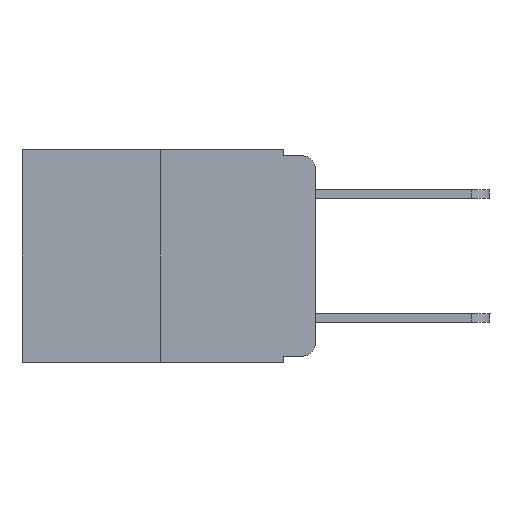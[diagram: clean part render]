
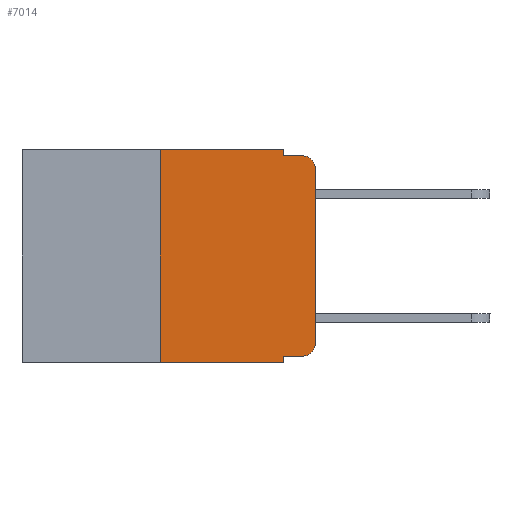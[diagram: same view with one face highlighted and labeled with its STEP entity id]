
A CAD part, left-side view. The second image highlights one B-rep face of the part: STEP entity #7014.
In plain terms, the highlighted planar face has unit normal (-1, 0, 0).
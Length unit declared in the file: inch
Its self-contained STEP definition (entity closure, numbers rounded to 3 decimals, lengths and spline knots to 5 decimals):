
#77 = DIRECTION ( 'NONE',  ( -1., 0., 0. ) ) ;
#237 = DIRECTION ( 'NONE',  ( 0., 0., -1. ) ) ;
#248 = VECTOR ( 'NONE', #7634, 39.37008 ) ;
#265 = ORIENTED_EDGE ( 'NONE', *, *, #8095, .T. ) ;
#505 = EDGE_CURVE ( 'NONE', #902, #5652, #4131, .T. ) ;
#508 = CARTESIAN_POINT ( 'NONE',  ( 0., 0.051, 0. ) ) ;
#626 = FACE_OUTER_BOUND ( 'NONE', #7078, .T. ) ;
#631 = CARTESIAN_POINT ( 'NONE',  ( 0., 0.051, -0.333 ) ) ;
#642 = DIRECTION ( 'NONE',  ( 0., -1., 0. ) ) ;
#769 = VECTOR ( 'NONE', #952, 39.37008 ) ;
#902 = VERTEX_POINT ( 'NONE', #631 ) ;
#952 = DIRECTION ( 'NONE',  ( 0., -1., 0. ) ) ;
#964 = CARTESIAN_POINT ( 'NONE',  ( 0., 0.02, -0.313 ) ) ;
#1249 = CARTESIAN_POINT ( 'NONE',  ( 0., 0.051, 0. ) ) ;
#1405 = VECTOR ( 'NONE', #2463, 39.37008 ) ;
#1528 = VERTEX_POINT ( 'NONE', #9574 ) ;
#1650 = DIRECTION ( 'NONE',  ( 0., 0., 1. ) ) ;
#2032 = DIRECTION ( 'NONE',  ( 0., 0., 1. ) ) ;
#2216 = CARTESIAN_POINT ( 'NONE',  ( 0., 0.02, -0.333 ) ) ;
#2238 = VERTEX_POINT ( 'NONE', #9872 ) ;
#2241 = PLANE ( 'NONE',  #5627 ) ;
#2316 = LINE ( 'NONE', #2430, #7866 ) ;
#2335 = DIRECTION ( 'NONE',  ( 0., 0., -1. ) ) ;
#2430 = CARTESIAN_POINT ( 'NONE',  ( 0., 0.25, 0. ) ) ;
#2463 = DIRECTION ( 'NONE',  ( 0., 0., -1. ) ) ;
#2515 = DIRECTION ( 'NONE',  ( -1., 0., 0. ) ) ;
#2792 = LINE ( 'NONE', #9548, #10254 ) ;
#2938 = EDGE_CURVE ( 'NONE', #10336, #5349, #10252, .T. ) ;
#3076 = CARTESIAN_POINT ( 'NONE',  ( 0., 0.051, -0.333 ) ) ;
#3347 = LINE ( 'NONE', #8389, #1405 ) ;
#3853 = CARTESIAN_POINT ( 'NONE',  ( 0., 0., -0.03 ) ) ;
#3881 = CARTESIAN_POINT ( 'NONE',  ( 0., 0.051, -0.01 ) ) ;
#3893 = EDGE_CURVE ( 'NONE', #2238, #1528, #5090, .T. ) ;
#3958 = ORIENTED_EDGE ( 'NONE', *, *, #505, .T. ) ;
#4035 = VERTEX_POINT ( 'NONE', #8278 ) ;
#4131 = LINE ( 'NONE', #3076, #8158 ) ;
#4866 = ORIENTED_EDGE ( 'NONE', *, *, #8344, .T. ) ;
#5069 = DIRECTION ( 'NONE',  ( 0., 0., -1. ) ) ;
#5090 = LINE ( 'NONE', #8459, #248 ) ;
#5250 = CIRCLE ( 'NONE', #6502, 0.02 ) ;
#5269 = ORIENTED_EDGE ( 'NONE', *, *, #2938, .F. ) ;
#5349 = VERTEX_POINT ( 'NONE', #8251 ) ;
#5374 = VECTOR ( 'NONE', #9666, 39.37008 ) ;
#5627 = AXIS2_PLACEMENT_3D ( 'NONE', #10646, #9917, #2335 ) ;
#5652 = VERTEX_POINT ( 'NONE', #2216 ) ;
#5682 = CARTESIAN_POINT ( 'NONE',  ( 0., 0.473, 0. ) ) ;
#5722 = EDGE_CURVE ( 'NONE', #2238, #4035, #2316, .T. ) ;
#5774 = VERTEX_POINT ( 'NONE', #10004 ) ;
#5840 = CARTESIAN_POINT ( 'NONE',  ( 0., 0.02, -0.03 ) ) ;
#6225 = ORIENTED_EDGE ( 'NONE', *, *, #9552, .F. ) ;
#6317 = EDGE_CURVE ( 'NONE', #10433, #10336, #3347, .T. ) ;
#6472 = LINE ( 'NONE', #5682, #6982 ) ;
#6502 = AXIS2_PLACEMENT_3D ( 'NONE', #5840, #2515, #5069 ) ;
#6982 = VECTOR ( 'NONE', #642, 39.37008 ) ;
#7014 = ADVANCED_FACE ( 'NONE', ( #626 ), #2241, .F. ) ;
#7078 = EDGE_LOOP ( 'NONE', ( #265, #4866, #5269, #9723, #6225, #9231, #7219, #8870, #3958, #10761 ) ) ;
#7219 = ORIENTED_EDGE ( 'NONE', *, *, #3893, .T. ) ;
#7634 = DIRECTION ( 'NONE',  ( 0., -1., 0. ) ) ;
#7762 = CARTESIAN_POINT ( 'NONE',  ( 0., 0.051, -0.01 ) ) ;
#7866 = VECTOR ( 'NONE', #1650, 39.37008 ) ;
#8095 = EDGE_CURVE ( 'NONE', #5774, #9568, #2792, .T. ) ;
#8158 = VECTOR ( 'NONE', #10617, 39.37008 ) ;
#8172 = CIRCLE ( 'NONE', #8551, 0.02 ) ;
#8251 = CARTESIAN_POINT ( 'NONE',  ( 0., 0.02, -0.01 ) ) ;
#8278 = CARTESIAN_POINT ( 'NONE',  ( 0., 0.25, 0. ) ) ;
#8344 = EDGE_CURVE ( 'NONE', #9568, #5349, #5250, .T. ) ;
#8389 = CARTESIAN_POINT ( 'NONE',  ( 0., 0.051, 0. ) ) ;
#8459 = CARTESIAN_POINT ( 'NONE',  ( 0., 0.473, -0.343 ) ) ;
#8551 = AXIS2_PLACEMENT_3D ( 'NONE', #964, #77, #237 ) ;
#8870 = ORIENTED_EDGE ( 'NONE', *, *, #9578, .F. ) ;
#9231 = ORIENTED_EDGE ( 'NONE', *, *, #5722, .F. ) ;
#9548 = CARTESIAN_POINT ( 'NONE',  ( 0., 0., 0. ) ) ;
#9552 = EDGE_CURVE ( 'NONE', #4035, #10433, #6472, .T. ) ;
#9568 = VERTEX_POINT ( 'NONE', #3853 ) ;
#9574 = CARTESIAN_POINT ( 'NONE',  ( 0., 0.051, -0.343 ) ) ;
#9578 = EDGE_CURVE ( 'NONE', #902, #1528, #9770, .T. ) ;
#9666 = DIRECTION ( 'NONE',  ( 0., 0., -1. ) ) ;
#9723 = ORIENTED_EDGE ( 'NONE', *, *, #6317, .F. ) ;
#9770 = LINE ( 'NONE', #1249, #5374 ) ;
#9773 = EDGE_CURVE ( 'NONE', #5652, #5774, #8172, .T. ) ;
#9872 = CARTESIAN_POINT ( 'NONE',  ( 0., 0.25, -0.343 ) ) ;
#9917 = DIRECTION ( 'NONE',  ( 1., 0., 0. ) ) ;
#10004 = CARTESIAN_POINT ( 'NONE',  ( 0., 0., -0.313 ) ) ;
#10252 = LINE ( 'NONE', #7762, #769 ) ;
#10254 = VECTOR ( 'NONE', #2032, 39.37008 ) ;
#10336 = VERTEX_POINT ( 'NONE', #3881 ) ;
#10433 = VERTEX_POINT ( 'NONE', #508 ) ;
#10617 = DIRECTION ( 'NONE',  ( 0., -1., 0. ) ) ;
#10646 = CARTESIAN_POINT ( 'NONE',  ( 0., 0.473, 0. ) ) ;
#10761 = ORIENTED_EDGE ( 'NONE', *, *, #9773, .T. ) ;
